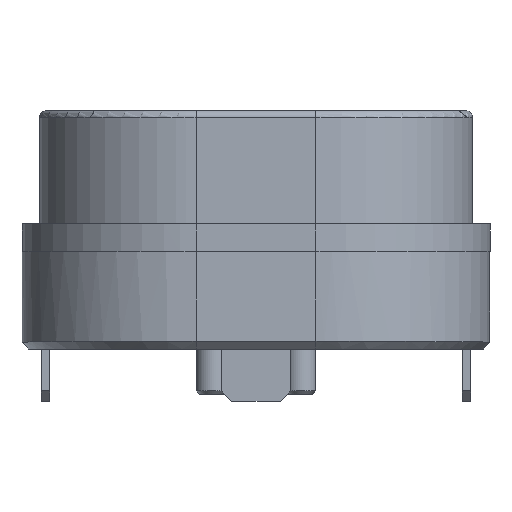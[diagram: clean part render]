
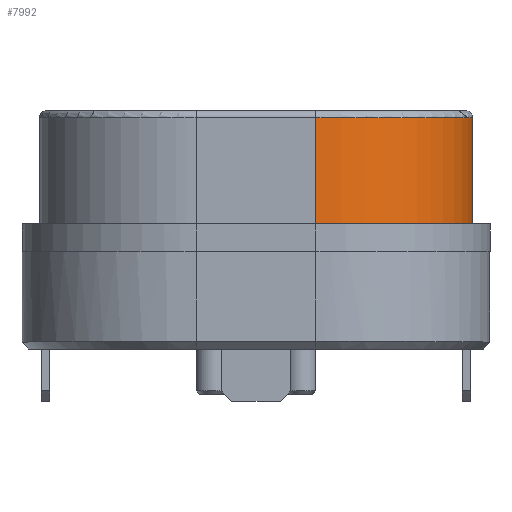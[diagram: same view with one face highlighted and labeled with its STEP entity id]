
A CAD part, left-side view. The second image highlights one B-rep face of the part: STEP entity #7992.
In plain terms, the highlighted cylindrical face has radius 4.5 mm (diameter 9 mm), a partial arc.
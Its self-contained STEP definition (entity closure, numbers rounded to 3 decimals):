
#50 = B_SPLINE_CURVE_WITH_KNOTS ( 'NONE', 3,
 ( #19298, #22546, #11563, #2430, #15317, #36588, #11325, #10128, #8066, #6392 ),
 .UNSPECIFIED., .F., .F.,
 ( 4, 2, 2, 2, 4 ),
 ( 0., 0.25, 0.5, 0.75, 1. ),
 .UNSPECIFIED. ) ;
#1647 = CARTESIAN_POINT ( 'NONE',  ( -162.789, -104.485, 0. ) ) ;
#2430 = CARTESIAN_POINT ( 'NONE',  ( -163.122, -103.986, -3.05 ) ) ;
#6235 = DIRECTION ( 'NONE',  ( 1., 0., 0. ) ) ;
#6392 = CARTESIAN_POINT ( 'NONE',  ( -159.19, -106.22, -3.05 ) ) ;
#7583 = FACE_OUTER_BOUND ( 'NONE', #32768, .T. ) ;
#7992 = ADVANCED_FACE ( 'NONE', ( #7583 ), #42902, .T. ) ;
#8066 = CARTESIAN_POINT ( 'NONE',  ( -159.779, -106.22, -3.05 ) ) ;
#8420 = CARTESIAN_POINT ( 'NONE',  ( -163.69, -101.72, -2.033 ) ) ;
#8847 = CARTESIAN_POINT ( 'NONE',  ( -163.69, -101.72, 0. ) ) ;
#9341 = CARTESIAN_POINT ( 'NONE',  ( -159.19, -106.22, 0. ) ) ;
#10128 = CARTESIAN_POINT ( 'NONE',  ( -160.368, -106.103, -3.05 ) ) ;
#11325 = CARTESIAN_POINT ( 'NONE',  ( -161.456, -105.652, -3.05 ) ) ;
#11563 = CARTESIAN_POINT ( 'NONE',  ( -163.573, -102.898, -3.05 ) ) ;
#13076 = CARTESIAN_POINT ( 'NONE',  ( -161.456, -105.652, 0. ) ) ;
#13707 = CARTESIAN_POINT ( 'NONE',  ( -159.19, -106.22, -3.05 ) ) ;
#15097 = CARTESIAN_POINT ( 'NONE',  ( -159.19, -106.22, 0. ) ) ;
#15317 = CARTESIAN_POINT ( 'NONE',  ( -162.789, -104.485, -3.05 ) ) ;
#16146 = EDGE_CURVE ( 'NONE', #34909, #17958, #46638, .T. ) ;
#17448 = B_SPLINE_CURVE_WITH_KNOTS ( 'NONE', 3,
 ( #8847, #46982, #31982, #20583, #1647, #47211, #13076, #28258, #43480, #9341 ),
 .UNSPECIFIED., .F., .F.,
 ( 4, 2, 2, 2, 4 ),
 ( 0., 0.25, 0.5, 0.75, 1. ),
 .UNSPECIFIED. ) ;
#17958 = VERTEX_POINT ( 'NONE', #15097 ) ;
#19298 = CARTESIAN_POINT ( 'NONE',  ( -163.69, -101.72, -3.05 ) ) ;
#20583 = CARTESIAN_POINT ( 'NONE',  ( -163.122, -103.986, 0. ) ) ;
#20716 = B_SPLINE_CURVE_WITH_KNOTS ( 'NONE', 3,
 ( #30832, #46044, #8420, #35341 ),
 .UNSPECIFIED., .F., .F.,
 ( 4, 4 ),
 ( 0., 1. ),
 .UNSPECIFIED. ) ;
#22546 = CARTESIAN_POINT ( 'NONE',  ( -163.69, -102.309, -3.05 ) ) ;
#24714 = EDGE_CURVE ( 'NONE', #43283, #48636, #20716, .T. ) ;
#26604 = CARTESIAN_POINT ( 'NONE',  ( -159.19, -106.22, 0. ) ) ;
#27704 = CARTESIAN_POINT ( 'NONE',  ( -163.69, -101.72, 0. ) ) ;
#28258 = CARTESIAN_POINT ( 'NONE',  ( -160.368, -106.103, 0. ) ) ;
#28372 = CARTESIAN_POINT ( 'NONE',  ( -163.69, -101.72, -3.05 ) ) ;
#30105 = CARTESIAN_POINT ( 'NONE',  ( -159.19, -106.22, -2.033 ) ) ;
#30832 = CARTESIAN_POINT ( 'NONE',  ( -163.69, -101.72, 0. ) ) ;
#31982 = CARTESIAN_POINT ( 'NONE',  ( -163.573, -102.898, 0. ) ) ;
#32768 = EDGE_LOOP ( 'NONE', ( #43455, #34512, #40780, #36673 ) ) ;
#33961 = EDGE_CURVE ( 'NONE', #43283, #17958, #17448, .T. ) ;
#34512 = ORIENTED_EDGE ( 'NONE', *, *, #33961, .F. ) ;
#34909 = VERTEX_POINT ( 'NONE', #13707 ) ;
#35341 = CARTESIAN_POINT ( 'NONE',  ( -163.69, -101.72, -3.05 ) ) ;
#36588 = CARTESIAN_POINT ( 'NONE',  ( -161.955, -105.319, -3.05 ) ) ;
#36673 = ORIENTED_EDGE ( 'NONE', *, *, #48924, .T. ) ;
#36808 = AXIS2_PLACEMENT_3D ( 'NONE', #40392, #44107, #6235 ) ;
#40392 = CARTESIAN_POINT ( 'NONE',  ( -159.19, -101.72, -3.111 ) ) ;
#40780 = ORIENTED_EDGE ( 'NONE', *, *, #24714, .T. ) ;
#42082 = CARTESIAN_POINT ( 'NONE',  ( -159.19, -106.22, -3.05 ) ) ;
#42902 = CYLINDRICAL_SURFACE ( 'NONE', #36808, 4.5 ) ;
#43283 = VERTEX_POINT ( 'NONE', #27704 ) ;
#43455 = ORIENTED_EDGE ( 'NONE', *, *, #16146, .T. ) ;
#43480 = CARTESIAN_POINT ( 'NONE',  ( -159.779, -106.22, 0. ) ) ;
#44107 = DIRECTION ( 'NONE',  ( 0., 0., 1. ) ) ;
#45329 = CARTESIAN_POINT ( 'NONE',  ( -159.19, -106.22, -1.017 ) ) ;
#46044 = CARTESIAN_POINT ( 'NONE',  ( -163.69, -101.72, -1.017 ) ) ;
#46638 = B_SPLINE_CURVE_WITH_KNOTS ( 'NONE', 3,
 ( #42082, #30105, #45329, #26604 ),
 .UNSPECIFIED., .F., .F.,
 ( 4, 4 ),
 ( 0., 1. ),
 .UNSPECIFIED. ) ;
#46982 = CARTESIAN_POINT ( 'NONE',  ( -163.69, -102.309, 0. ) ) ;
#47211 = CARTESIAN_POINT ( 'NONE',  ( -161.955, -105.319, 0. ) ) ;
#48636 = VERTEX_POINT ( 'NONE', #28372 ) ;
#48924 = EDGE_CURVE ( 'NONE', #48636, #34909, #50, .T. ) ;
